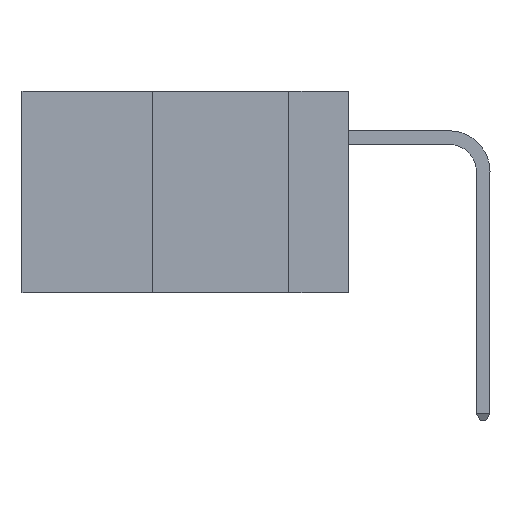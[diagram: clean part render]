
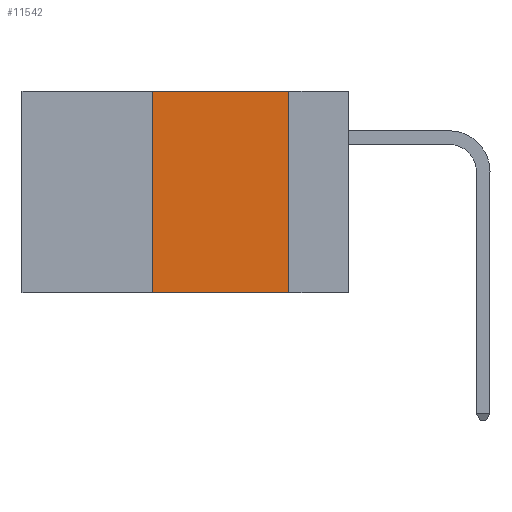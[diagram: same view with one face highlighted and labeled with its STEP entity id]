
A CAD part, left-side view. The second image highlights one B-rep face of the part: STEP entity #11542.
In plain terms, the highlighted planar face has unit normal (-1, 0, 0).
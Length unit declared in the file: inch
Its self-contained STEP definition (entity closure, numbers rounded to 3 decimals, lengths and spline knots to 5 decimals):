
#1100 = DIRECTION ( 'NONE',  ( 0., 0., 1. ) ) ;
#1509 = ORIENTED_EDGE ( 'NONE', *, *, #4527, .F. ) ;
#2005 = FACE_OUTER_BOUND ( 'NONE', #9905, .T. ) ;
#2931 = VECTOR ( 'NONE', #14235, 39.37008 ) ;
#3031 = EDGE_CURVE ( 'NONE', #8534, #13251, #7315, .T. ) ;
#3059 = DIRECTION ( 'NONE',  ( 1., 0., 0. ) ) ;
#4527 = EDGE_CURVE ( 'NONE', #13251, #9646, #5145, .T. ) ;
#5105 = EDGE_CURVE ( 'NONE', #6835, #8534, #15616, .T. ) ;
#5145 = LINE ( 'NONE', #6174, #11557 ) ;
#5835 = CARTESIAN_POINT ( 'NONE',  ( 0., 0.6, 0. ) ) ;
#6174 = CARTESIAN_POINT ( 'NONE',  ( 0., 0.11, 0. ) ) ;
#6187 = CARTESIAN_POINT ( 'NONE',  ( 0., 0.6, -0.37 ) ) ;
#6456 = VECTOR ( 'NONE', #1100, 39.37008 ) ;
#6539 = VECTOR ( 'NONE', #7388, 39.37008 ) ;
#6835 = VERTEX_POINT ( 'NONE', #13520 ) ;
#7315 = LINE ( 'NONE', #5835, #2931 ) ;
#7388 = DIRECTION ( 'NONE',  ( 0., -1., 0. ) ) ;
#7991 = ORIENTED_EDGE ( 'NONE', *, *, #3031, .F. ) ;
#8534 = VERTEX_POINT ( 'NONE', #10891 ) ;
#8896 = CARTESIAN_POINT ( 'NONE',  ( 0., 0.11, 0. ) ) ;
#9103 = PLANE ( 'NONE',  #11349 ) ;
#9646 = VERTEX_POINT ( 'NONE', #13029 ) ;
#9905 = EDGE_LOOP ( 'NONE', ( #1509, #7991, #14379, #15466 ) ) ;
#10114 = LINE ( 'NONE', #6187, #6539 ) ;
#10305 = CARTESIAN_POINT ( 'NONE',  ( 0., 0.6, 0. ) ) ;
#10891 = CARTESIAN_POINT ( 'NONE',  ( 0., 0.36, 0. ) ) ;
#11349 = AXIS2_PLACEMENT_3D ( 'NONE', #10305, #3059, #11514 ) ;
#11514 = DIRECTION ( 'NONE',  ( 0., 0., -1. ) ) ;
#11542 = ADVANCED_FACE ( 'NONE', ( #2005 ), #9103, .F. ) ;
#11557 = VECTOR ( 'NONE', #14547, 39.37008 ) ;
#12567 = EDGE_CURVE ( 'NONE', #6835, #9646, #10114, .T. ) ;
#13029 = CARTESIAN_POINT ( 'NONE',  ( 0., 0.11, -0.37 ) ) ;
#13251 = VERTEX_POINT ( 'NONE', #8896 ) ;
#13520 = CARTESIAN_POINT ( 'NONE',  ( 0., 0.36, -0.37 ) ) ;
#14235 = DIRECTION ( 'NONE',  ( 0., -1., 0. ) ) ;
#14379 = ORIENTED_EDGE ( 'NONE', *, *, #5105, .F. ) ;
#14547 = DIRECTION ( 'NONE',  ( 0., 0., -1. ) ) ;
#15466 = ORIENTED_EDGE ( 'NONE', *, *, #12567, .T. ) ;
#15554 = CARTESIAN_POINT ( 'NONE',  ( 0., 0.36, 0. ) ) ;
#15616 = LINE ( 'NONE', #15554, #6456 ) ;
